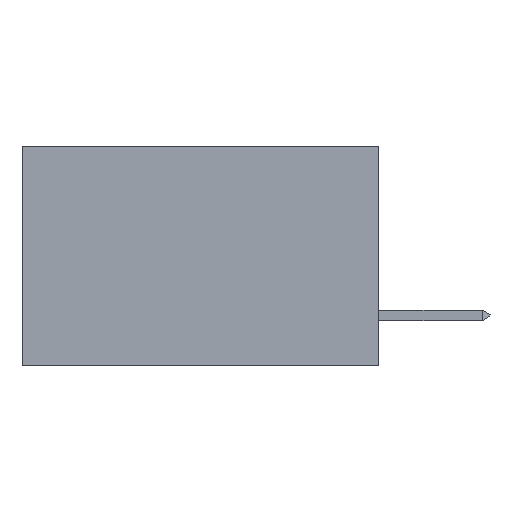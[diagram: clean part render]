
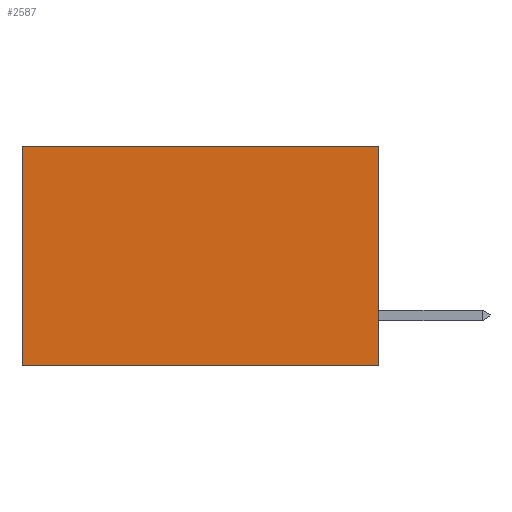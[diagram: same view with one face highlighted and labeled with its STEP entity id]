
A CAD part, left-side view. The second image highlights one B-rep face of the part: STEP entity #2587.
In plain terms, the highlighted planar face has unit normal (-1, 0, 0).
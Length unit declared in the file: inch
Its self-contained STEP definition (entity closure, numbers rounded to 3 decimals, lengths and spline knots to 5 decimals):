
#309 = EDGE_LOOP ( 'NONE', ( #404, #9759, #1363, #4870 ) ) ;
#404 = ORIENTED_EDGE ( 'NONE', *, *, #1227, .T. ) ;
#445 = EDGE_CURVE ( 'NONE', #8970, #2237, #1430, .T. ) ;
#644 = EDGE_CURVE ( 'NONE', #3745, #3051, #7638, .T. ) ;
#958 = VECTOR ( 'NONE', #4625, 39.37008 ) ;
#1081 = CARTESIAN_POINT ( 'NONE',  ( 0.2615, 0., -0.37 ) ) ;
#1227 = EDGE_CURVE ( 'NONE', #2237, #3051, #3559, .T. ) ;
#1237 = CARTESIAN_POINT ( 'NONE',  ( 0.2615, 0.6, -0.37 ) ) ;
#1363 = ORIENTED_EDGE ( 'NONE', *, *, #6219, .F. ) ;
#1430 = LINE ( 'NONE', #9276, #5076 ) ;
#2044 = CARTESIAN_POINT ( 'NONE',  ( 0.2615, 0., -0.37 ) ) ;
#2237 = VERTEX_POINT ( 'NONE', #9683 ) ;
#2587 = ADVANCED_FACE ( 'NONE', ( #6014 ), #6162, .F. ) ;
#3051 = VERTEX_POINT ( 'NONE', #5332 ) ;
#3103 = VECTOR ( 'NONE', #3445, 39.37008 ) ;
#3445 = DIRECTION ( 'NONE',  ( 0., 0., -1. ) ) ;
#3497 = AXIS2_PLACEMENT_3D ( 'NONE', #3657, #3712, #9868 ) ;
#3559 = LINE ( 'NONE', #1237, #3103 ) ;
#3657 = CARTESIAN_POINT ( 'NONE',  ( 0.2615, 0., -0.37 ) ) ;
#3712 = DIRECTION ( 'NONE',  ( 1., 0., 0. ) ) ;
#3745 = VERTEX_POINT ( 'NONE', #1081 ) ;
#3880 = DIRECTION ( 'NONE',  ( 0., 1., 0. ) ) ;
#3941 = CARTESIAN_POINT ( 'NONE',  ( 0.2615, 0., -0.37 ) ) ;
#4625 = DIRECTION ( 'NONE',  ( 0., 1., 0. ) ) ;
#4870 = ORIENTED_EDGE ( 'NONE', *, *, #445, .T. ) ;
#5076 = VECTOR ( 'NONE', #3880, 39.37008 ) ;
#5332 = CARTESIAN_POINT ( 'NONE',  ( 0.2615, 0.6, -0.37 ) ) ;
#5374 = LINE ( 'NONE', #3941, #5996 ) ;
#5996 = VECTOR ( 'NONE', #8590, 39.37008 ) ;
#6014 = FACE_OUTER_BOUND ( 'NONE', #309, .T. ) ;
#6162 = PLANE ( 'NONE',  #3497 ) ;
#6219 = EDGE_CURVE ( 'NONE', #8970, #3745, #5374, .T. ) ;
#7638 = LINE ( 'NONE', #2044, #958 ) ;
#8590 = DIRECTION ( 'NONE',  ( 0., 0., -1. ) ) ;
#8970 = VERTEX_POINT ( 'NONE', #9330 ) ;
#9276 = CARTESIAN_POINT ( 'NONE',  ( 0.2615, 0., 0. ) ) ;
#9330 = CARTESIAN_POINT ( 'NONE',  ( 0.2615, 0., 0. ) ) ;
#9683 = CARTESIAN_POINT ( 'NONE',  ( 0.2615, 0.6, 0. ) ) ;
#9759 = ORIENTED_EDGE ( 'NONE', *, *, #644, .F. ) ;
#9868 = DIRECTION ( 'NONE',  ( 0., 0., -1. ) ) ;
